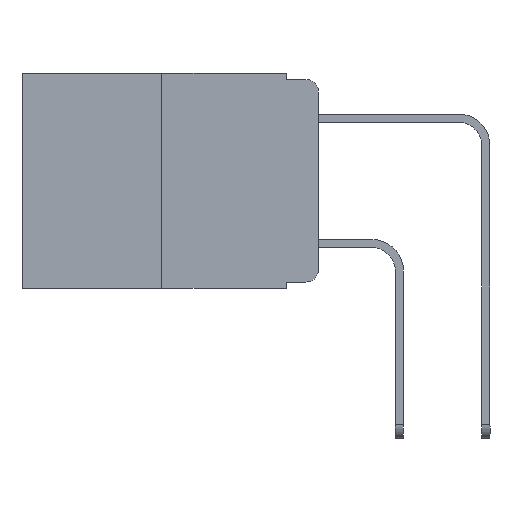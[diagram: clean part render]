
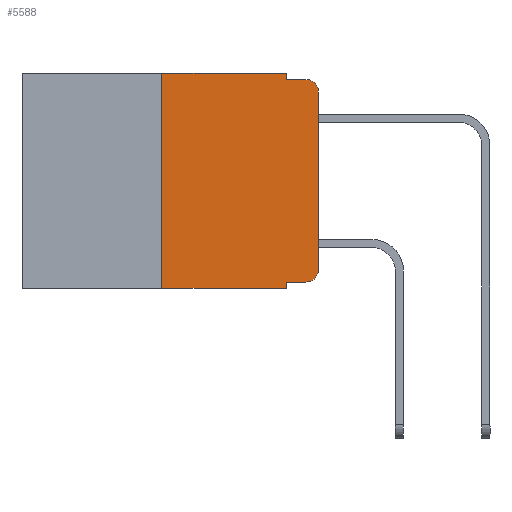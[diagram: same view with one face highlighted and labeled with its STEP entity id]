
A CAD part, left-side view. The second image highlights one B-rep face of the part: STEP entity #5588.
In plain terms, the highlighted planar face has unit normal (-1, 0, 0).
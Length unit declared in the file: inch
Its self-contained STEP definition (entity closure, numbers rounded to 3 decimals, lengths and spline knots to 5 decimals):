
#31 = LINE ( 'NONE', #8111, #9051 ) ;
#192 = DIRECTION ( 'NONE',  ( 0., 0., -1. ) ) ;
#208 = VECTOR ( 'NONE', #8815, 39.37008 ) ;
#232 = EDGE_CURVE ( 'NONE', #6879, #10117, #13310, .T. ) ;
#538 = ORIENTED_EDGE ( 'NONE', *, *, #12976, .F. ) ;
#590 = CARTESIAN_POINT ( 'NONE',  ( 0., 0.473, -0.343 ) ) ;
#957 = VERTEX_POINT ( 'NONE', #4366 ) ;
#1028 = DIRECTION ( 'NONE',  ( 0., -1., 0. ) ) ;
#1063 = VECTOR ( 'NONE', #10114, 39.37008 ) ;
#1426 = DIRECTION ( 'NONE',  ( 0., 0., 1. ) ) ;
#1548 = ORIENTED_EDGE ( 'NONE', *, *, #8767, .T. ) ;
#1587 = EDGE_CURVE ( 'NONE', #957, #7821, #8521, .T. ) ;
#1780 = VECTOR ( 'NONE', #8595, 39.37008 ) ;
#2053 = ORIENTED_EDGE ( 'NONE', *, *, #3673, .F. ) ;
#2214 = CARTESIAN_POINT ( 'NONE',  ( 0., 0.051, 0. ) ) ;
#2566 = DIRECTION ( 'NONE',  ( 0., 0., -1. ) ) ;
#2708 = CARTESIAN_POINT ( 'NONE',  ( 0., 0.473, 0. ) ) ;
#3491 = CARTESIAN_POINT ( 'NONE',  ( 0., 0.25, 0. ) ) ;
#3555 = CARTESIAN_POINT ( 'NONE',  ( 0., 0., 0. ) ) ;
#3673 = EDGE_CURVE ( 'NONE', #6216, #6656, #31, .T. ) ;
#3704 = LINE ( 'NONE', #12935, #3864 ) ;
#3817 = VECTOR ( 'NONE', #1028, 39.37008 ) ;
#3864 = VECTOR ( 'NONE', #12856, 39.37008 ) ;
#4044 = CARTESIAN_POINT ( 'NONE',  ( 0., 0.02, -0.03 ) ) ;
#4107 = DIRECTION ( 'NONE',  ( -1., 0., 0. ) ) ;
#4366 = CARTESIAN_POINT ( 'NONE',  ( 0., 0.051, -0.333 ) ) ;
#4844 = DIRECTION ( 'NONE',  ( 1., 0., 0. ) ) ;
#4960 = CARTESIAN_POINT ( 'NONE',  ( 0., 0.051, -0.343 ) ) ;
#5318 = VECTOR ( 'NONE', #1426, 39.37008 ) ;
#5439 = EDGE_CURVE ( 'NONE', #9612, #6216, #11708, .T. ) ;
#5588 = ADVANCED_FACE ( 'NONE', ( #7270 ), #9773, .F. ) ;
#6006 = LINE ( 'NONE', #3555, #5318 ) ;
#6020 = CARTESIAN_POINT ( 'NONE',  ( 0., 0.02, -0.333 ) ) ;
#6047 = DIRECTION ( 'NONE',  ( -1., 0., 0. ) ) ;
#6094 = CARTESIAN_POINT ( 'NONE',  ( 0., 0.25, 0. ) ) ;
#6102 = DIRECTION ( 'NONE',  ( 0., -1., 0. ) ) ;
#6216 = VERTEX_POINT ( 'NONE', #2214 ) ;
#6315 = CARTESIAN_POINT ( 'NONE',  ( 0., 0.051, -0.01 ) ) ;
#6623 = EDGE_CURVE ( 'NONE', #7431, #7821, #9878, .T. ) ;
#6656 = VERTEX_POINT ( 'NONE', #6315 ) ;
#6736 = ORIENTED_EDGE ( 'NONE', *, *, #6851, .T. ) ;
#6851 = EDGE_CURVE ( 'NONE', #13044, #6879, #6006, .T. ) ;
#6879 = VERTEX_POINT ( 'NONE', #10488 ) ;
#7026 = ORIENTED_EDGE ( 'NONE', *, *, #6623, .T. ) ;
#7270 = FACE_OUTER_BOUND ( 'NONE', #9327, .T. ) ;
#7431 = VERTEX_POINT ( 'NONE', #11057 ) ;
#7492 = ORIENTED_EDGE ( 'NONE', *, *, #232, .T. ) ;
#7749 = EDGE_CURVE ( 'NONE', #6656, #10117, #15008, .T. ) ;
#7821 = VERTEX_POINT ( 'NONE', #4960 ) ;
#7894 = LINE ( 'NONE', #3491, #1063 ) ;
#8111 = CARTESIAN_POINT ( 'NONE',  ( 0., 0.051, 0. ) ) ;
#8521 = LINE ( 'NONE', #8740, #1780 ) ;
#8552 = CIRCLE ( 'NONE', #8788, 0.02 ) ;
#8595 = DIRECTION ( 'NONE',  ( 0., 0., -1. ) ) ;
#8740 = CARTESIAN_POINT ( 'NONE',  ( 0., 0.051, 0. ) ) ;
#8767 = EDGE_CURVE ( 'NONE', #957, #11363, #3704, .T. ) ;
#8788 = AXIS2_PLACEMENT_3D ( 'NONE', #9895, #4107, #13420 ) ;
#8815 = DIRECTION ( 'NONE',  ( 0., -1., 0. ) ) ;
#8868 = CARTESIAN_POINT ( 'NONE',  ( 0., 0.02, -0.01 ) ) ;
#8928 = ORIENTED_EDGE ( 'NONE', *, *, #5439, .F. ) ;
#9051 = VECTOR ( 'NONE', #192, 39.37008 ) ;
#9194 = VECTOR ( 'NONE', #6102, 39.37008 ) ;
#9327 = EDGE_LOOP ( 'NONE', ( #6736, #7492, #10653, #2053, #8928, #538, #7026, #11992, #1548, #9338 ) ) ;
#9338 = ORIENTED_EDGE ( 'NONE', *, *, #11098, .T. ) ;
#9428 = CARTESIAN_POINT ( 'NONE',  ( 0., 0., -0.313 ) ) ;
#9612 = VERTEX_POINT ( 'NONE', #6094 ) ;
#9773 = PLANE ( 'NONE',  #14079 ) ;
#9878 = LINE ( 'NONE', #590, #208 ) ;
#9895 = CARTESIAN_POINT ( 'NONE',  ( 0., 0.02, -0.313 ) ) ;
#10114 = DIRECTION ( 'NONE',  ( 0., 0., 1. ) ) ;
#10117 = VERTEX_POINT ( 'NONE', #8868 ) ;
#10488 = CARTESIAN_POINT ( 'NONE',  ( 0., 0., -0.03 ) ) ;
#10653 = ORIENTED_EDGE ( 'NONE', *, *, #7749, .F. ) ;
#11057 = CARTESIAN_POINT ( 'NONE',  ( 0., 0.25, -0.343 ) ) ;
#11098 = EDGE_CURVE ( 'NONE', #11363, #13044, #8552, .T. ) ;
#11363 = VERTEX_POINT ( 'NONE', #6020 ) ;
#11626 = CARTESIAN_POINT ( 'NONE',  ( 0., 0.473, 0. ) ) ;
#11708 = LINE ( 'NONE', #11626, #3817 ) ;
#11992 = ORIENTED_EDGE ( 'NONE', *, *, #1587, .F. ) ;
#12131 = DIRECTION ( 'NONE',  ( 0., 0., -1. ) ) ;
#12856 = DIRECTION ( 'NONE',  ( 0., -1., 0. ) ) ;
#12935 = CARTESIAN_POINT ( 'NONE',  ( 0., 0.051, -0.333 ) ) ;
#12976 = EDGE_CURVE ( 'NONE', #7431, #9612, #7894, .T. ) ;
#13044 = VERTEX_POINT ( 'NONE', #9428 ) ;
#13310 = CIRCLE ( 'NONE', #13563, 0.02 ) ;
#13420 = DIRECTION ( 'NONE',  ( 0., 0., -1. ) ) ;
#13563 = AXIS2_PLACEMENT_3D ( 'NONE', #4044, #6047, #12131 ) ;
#14079 = AXIS2_PLACEMENT_3D ( 'NONE', #2708, #4844, #2566 ) ;
#14188 = CARTESIAN_POINT ( 'NONE',  ( 0., 0.051, -0.01 ) ) ;
#15008 = LINE ( 'NONE', #14188, #9194 ) ;
